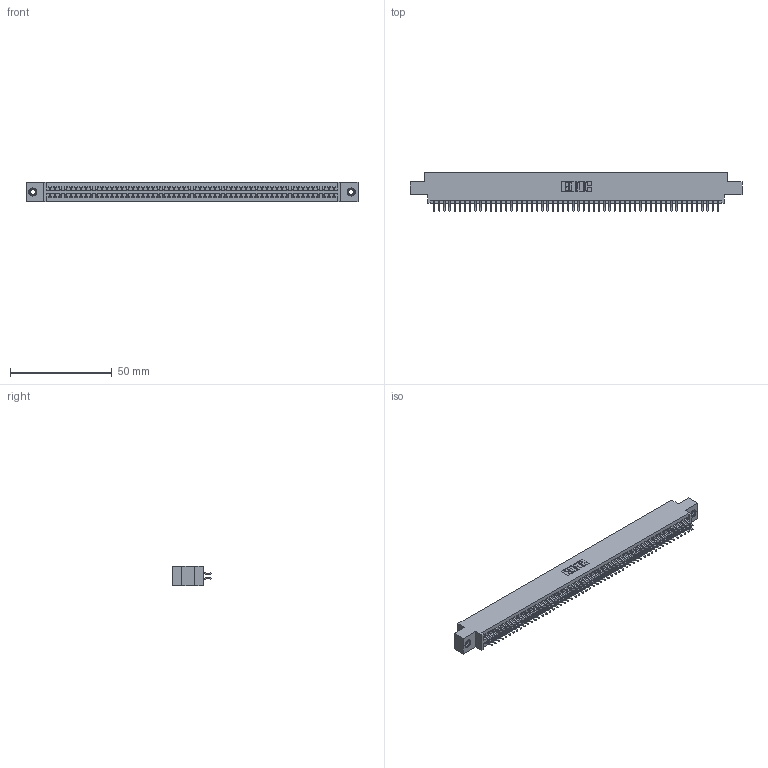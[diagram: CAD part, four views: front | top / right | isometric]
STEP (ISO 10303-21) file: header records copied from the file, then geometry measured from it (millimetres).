
FILE_DESCRIPTION (( 'STEP AP203' ), '1' );
FILE_NAME ('395-112-556-807.STEP', '2019-10-27T16:12:00', ( '' ), ( '' ), 'SwSTEP 2.0', 'SolidWorks 2016', '' );
FILE_SCHEMA (( 'CONFIG_CONTROL_DESIGN' ));
Length unit declared in the file: inch
Products named in the file (4): 345 Part_0.170 Offset - 0.156 Dia-TI; 345-292-001_556 Tail; 345-250-001_345-250-005-103; 395-112-556-807
Assembly tree (115 placements, depth 2):
  395-112-556-807
    345 Part_0.170 Offset - 0.156 Dia-TI
    345-292-001_556 Tail  x112
    345-250-001_345-250-005-103  x2
Bounding box: 163.45 x 19.24 x 9.4 mm (x, y, z)
Volume: 15876.2 mm3; surface area: 23812.2 mm2
Topology: 115 solids, 115 shells, 6462 faces, 19193 edges, 12638 vertices
Faces by surface type: plane 4260, cylinder 2186, cone 12, torus 4
Entity records: 43592 total; most frequent: CARTESIAN_POINT 7291, ORIENTED_EDGE 7206, DIRECTION 6425, EDGE_CURVE 3603, VECTOR 3219, LINE 3219, VERTEX_POINT 2396, AXIS2_PLACEMENT_3D 1603
